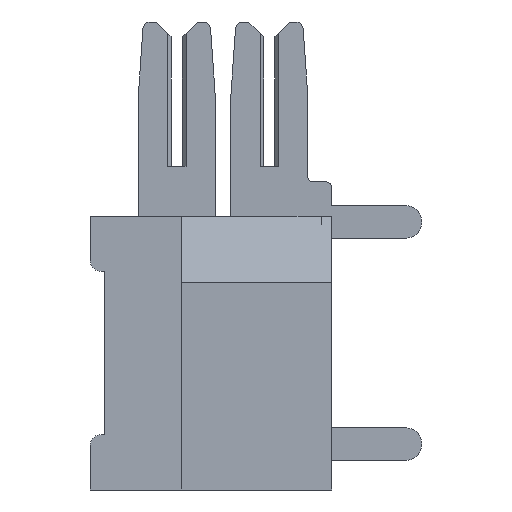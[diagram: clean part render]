
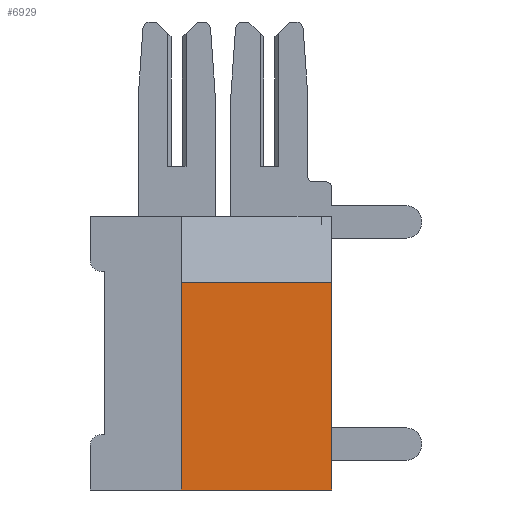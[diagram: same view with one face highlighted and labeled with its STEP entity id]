
A CAD part, left-side view. The second image highlights one B-rep face of the part: STEP entity #6929.
In plain terms, the highlighted planar face has unit normal (-1, 0, 0).
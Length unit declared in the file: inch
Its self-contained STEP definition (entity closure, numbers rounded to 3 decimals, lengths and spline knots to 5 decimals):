
#3 = DIRECTION ( 'NONE',  ( 0., 0., 1. ) ) ;
#194 = AXIS2_PLACEMENT_3D ( 'NONE', #5432, #6158, #1806 ) ;
#460 = CARTESIAN_POINT ( 'NONE',  ( 0., 0., 0. ) ) ;
#483 = VECTOR ( 'NONE', #2227, 39.37008 ) ;
#635 = EDGE_CURVE ( 'NONE', #6693, #5589, #2459, .T. ) ;
#719 = FACE_OUTER_BOUND ( 'NONE', #6541, .T. ) ;
#1489 = LINE ( 'NONE', #3670, #483 ) ;
#1806 = DIRECTION ( 'NONE',  ( 0., 0., -1. ) ) ;
#2227 = DIRECTION ( 'NONE',  ( 0., -1., 0. ) ) ;
#2459 = LINE ( 'NONE', #3601, #3481 ) ;
#2538 = PLANE ( 'NONE',  #194 ) ;
#3120 = ORIENTED_EDGE ( 'NONE', *, *, #635, .T. ) ;
#3183 = EDGE_CURVE ( 'NONE', #8973, #8325, #1489, .T. ) ;
#3481 = VECTOR ( 'NONE', #7230, 39.37008 ) ;
#3601 = CARTESIAN_POINT ( 'NONE',  ( 0., 0., -0.09 ) ) ;
#3670 = CARTESIAN_POINT ( 'NONE',  ( 0., 0.326, -0.37 ) ) ;
#3884 = ORIENTED_EDGE ( 'NONE', *, *, #3183, .T. ) ;
#4657 = CARTESIAN_POINT ( 'NONE',  ( 0., 0., -0.37 ) ) ;
#5432 = CARTESIAN_POINT ( 'NONE',  ( 0., 0.326, 0. ) ) ;
#5589 = VERTEX_POINT ( 'NONE', #6802 ) ;
#5723 = CARTESIAN_POINT ( 'NONE',  ( 0., 0.203, -0.37 ) ) ;
#5896 = LINE ( 'NONE', #5723, #7627 ) ;
#6094 = ORIENTED_EDGE ( 'NONE', *, *, #6762, .F. ) ;
#6158 = DIRECTION ( 'NONE',  ( 1., 0., 0. ) ) ;
#6393 = EDGE_CURVE ( 'NONE', #8325, #6693, #7851, .T. ) ;
#6541 = EDGE_LOOP ( 'NONE', ( #7003, #3120, #6094, #3884 ) ) ;
#6693 = VERTEX_POINT ( 'NONE', #7978 ) ;
#6762 = EDGE_CURVE ( 'NONE', #8973, #5589, #5896, .T. ) ;
#6802 = CARTESIAN_POINT ( 'NONE',  ( 0., 0.203, -0.09 ) ) ;
#6929 = ADVANCED_FACE ( 'NONE', ( #719 ), #2538, .F. ) ;
#7003 = ORIENTED_EDGE ( 'NONE', *, *, #6393, .T. ) ;
#7230 = DIRECTION ( 'NONE',  ( 0., 1., 0. ) ) ;
#7347 = CARTESIAN_POINT ( 'NONE',  ( 0., 0.203, -0.37 ) ) ;
#7627 = VECTOR ( 'NONE', #3, 39.37008 ) ;
#7851 = LINE ( 'NONE', #460, #8072 ) ;
#7978 = CARTESIAN_POINT ( 'NONE',  ( 0., 0., -0.09 ) ) ;
#8072 = VECTOR ( 'NONE', #9161, 39.37008 ) ;
#8325 = VERTEX_POINT ( 'NONE', #4657 ) ;
#8973 = VERTEX_POINT ( 'NONE', #7347 ) ;
#9161 = DIRECTION ( 'NONE',  ( 0., 0., 1. ) ) ;
